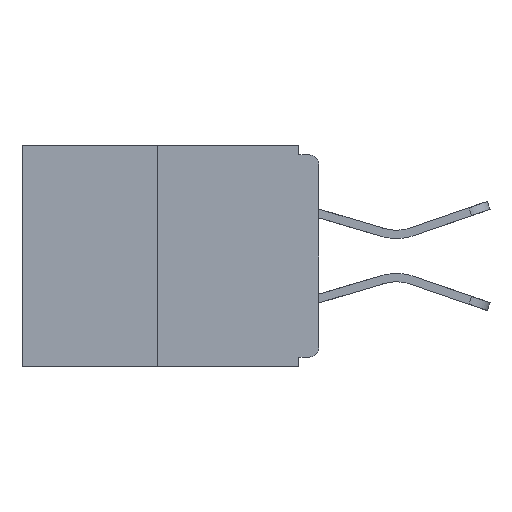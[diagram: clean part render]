
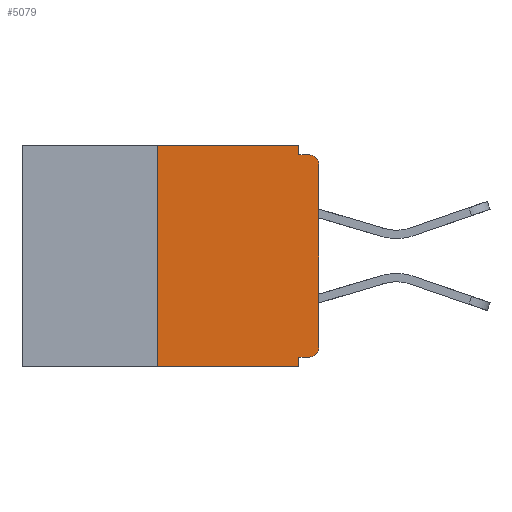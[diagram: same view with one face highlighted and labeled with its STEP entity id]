
A CAD part, left-side view. The second image highlights one B-rep face of the part: STEP entity #5079.
In plain terms, the highlighted planar face has unit normal (-1, 0, 0).
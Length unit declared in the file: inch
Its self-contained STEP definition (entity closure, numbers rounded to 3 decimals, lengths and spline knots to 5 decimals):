
#245 = DIRECTION ( 'NONE',  ( 1., 0., 0. ) ) ;
#256 = DIRECTION ( 'NONE',  ( -1., 0., 0. ) ) ;
#873 = VERTEX_POINT ( 'NONE', #2145 ) ;
#1524 = AXIS2_PLACEMENT_3D ( 'NONE', #5830, #245, #7463 ) ;
#1584 = LINE ( 'NONE', #21898, #17406 ) ;
#1611 = DIRECTION ( 'NONE',  ( 0., 0., 1. ) ) ;
#1694 = VERTEX_POINT ( 'NONE', #2825 ) ;
#2031 = CARTESIAN_POINT ( 'NONE',  ( 0., 0.015, -0.03 ) ) ;
#2145 = CARTESIAN_POINT ( 'NONE',  ( 0., 0., -0.03 ) ) ;
#2825 = CARTESIAN_POINT ( 'NONE',  ( 0., 0., -0.313 ) ) ;
#3088 = CARTESIAN_POINT ( 'NONE',  ( 0., 0.25, 0. ) ) ;
#3634 = VECTOR ( 'NONE', #22914, 39.37008 ) ;
#3731 = LINE ( 'NONE', #9060, #6418 ) ;
#3796 = EDGE_CURVE ( 'NONE', #4616, #9883, #1584, .T. ) ;
#3925 = PLANE ( 'NONE',  #1524 ) ;
#4080 = VECTOR ( 'NONE', #21179, 39.37008 ) ;
#4088 = VERTEX_POINT ( 'NONE', #3088 ) ;
#4372 = EDGE_CURVE ( 'NONE', #4088, #18091, #13389, .T. ) ;
#4557 = ORIENTED_EDGE ( 'NONE', *, *, #14546, .T. ) ;
#4616 = VERTEX_POINT ( 'NONE', #16344 ) ;
#4682 = AXIS2_PLACEMENT_3D ( 'NONE', #21091, #15497, #15159 ) ;
#4692 = DIRECTION ( 'NONE',  ( 0., -1., 0. ) ) ;
#4897 = CARTESIAN_POINT ( 'NONE',  ( 0., 0., 0. ) ) ;
#5079 = ADVANCED_FACE ( 'NONE', ( #19965 ), #3925, .F. ) ;
#5110 = CARTESIAN_POINT ( 'NONE',  ( 0., 0.031, 0. ) ) ;
#5830 = CARTESIAN_POINT ( 'NONE',  ( 0., 0.46, 0. ) ) ;
#6418 = VECTOR ( 'NONE', #1611, 39.37008 ) ;
#6474 = LINE ( 'NONE', #20983, #14541 ) ;
#6662 = CARTESIAN_POINT ( 'NONE',  ( 0., 0.015, -0.015 ) ) ;
#6881 = ORIENTED_EDGE ( 'NONE', *, *, #14597, .F. ) ;
#7301 = VECTOR ( 'NONE', #20868, 39.37008 ) ;
#7463 = DIRECTION ( 'NONE',  ( 0., 0., -1. ) ) ;
#7747 = VECTOR ( 'NONE', #17458, 39.37008 ) ;
#7790 = DIRECTION ( 'NONE',  ( 0., -1., 0. ) ) ;
#8229 = LINE ( 'NONE', #18727, #7301 ) ;
#8395 = CARTESIAN_POINT ( 'NONE',  ( 0., 0., -0.328 ) ) ;
#8791 = LINE ( 'NONE', #4897, #4080 ) ;
#9060 = CARTESIAN_POINT ( 'NONE',  ( 0., 0.25, 0. ) ) ;
#9267 = DIRECTION ( 'NONE',  ( 0., -1., 0. ) ) ;
#9642 = CARTESIAN_POINT ( 'NONE',  ( 0., 0.031, -0.343 ) ) ;
#9883 = VERTEX_POINT ( 'NONE', #9642 ) ;
#10383 = ORIENTED_EDGE ( 'NONE', *, *, #4372, .F. ) ;
#10672 = LINE ( 'NONE', #5110, #7747 ) ;
#10925 = DIRECTION ( 'NONE',  ( 0., 0., -1. ) ) ;
#10937 = EDGE_CURVE ( 'NONE', #4616, #4088, #3731, .T. ) ;
#11031 = AXIS2_PLACEMENT_3D ( 'NONE', #2031, #256, #10925 ) ;
#11621 = ORIENTED_EDGE ( 'NONE', *, *, #21747, .T. ) ;
#11745 = VERTEX_POINT ( 'NONE', #13734 ) ;
#12467 = EDGE_CURVE ( 'NONE', #873, #21868, #21676, .T. ) ;
#12709 = ORIENTED_EDGE ( 'NONE', *, *, #17196, .F. ) ;
#12951 = ORIENTED_EDGE ( 'NONE', *, *, #3796, .T. ) ;
#13389 = LINE ( 'NONE', #20652, #17081 ) ;
#13734 = CARTESIAN_POINT ( 'NONE',  ( 0., 0.031, -0.015 ) ) ;
#13936 = VERTEX_POINT ( 'NONE', #16734 ) ;
#14467 = EDGE_CURVE ( 'NONE', #17739, #9883, #8229, .T. ) ;
#14541 = VECTOR ( 'NONE', #4692, 39.37008 ) ;
#14546 = EDGE_CURVE ( 'NONE', #13936, #1694, #17572, .T. ) ;
#14597 = EDGE_CURVE ( 'NONE', #11745, #21868, #6474, .T. ) ;
#15159 = DIRECTION ( 'NONE',  ( 0., 0., -1. ) ) ;
#15497 = DIRECTION ( 'NONE',  ( -1., 0., 0. ) ) ;
#15771 = LINE ( 'NONE', #8395, #3634 ) ;
#15859 = ORIENTED_EDGE ( 'NONE', *, *, #18863, .F. ) ;
#16344 = CARTESIAN_POINT ( 'NONE',  ( 0., 0.25, -0.343 ) ) ;
#16734 = CARTESIAN_POINT ( 'NONE',  ( 0., 0.015, -0.328 ) ) ;
#17081 = VECTOR ( 'NONE', #7790, 39.37008 ) ;
#17196 = EDGE_CURVE ( 'NONE', #18091, #11745, #10672, .T. ) ;
#17404 = ORIENTED_EDGE ( 'NONE', *, *, #10937, .F. ) ;
#17406 = VECTOR ( 'NONE', #9267, 39.37008 ) ;
#17411 = CARTESIAN_POINT ( 'NONE',  ( 0., 0.031, 0. ) ) ;
#17458 = DIRECTION ( 'NONE',  ( 0., 0., -1. ) ) ;
#17572 = CIRCLE ( 'NONE', #4682, 0.015 ) ;
#17739 = VERTEX_POINT ( 'NONE', #19933 ) ;
#18091 = VERTEX_POINT ( 'NONE', #17411 ) ;
#18727 = CARTESIAN_POINT ( 'NONE',  ( 0., 0.031, -0.343 ) ) ;
#18863 = EDGE_CURVE ( 'NONE', #13936, #17739, #15771, .T. ) ;
#19933 = CARTESIAN_POINT ( 'NONE',  ( 0., 0.031, -0.328 ) ) ;
#19965 = FACE_OUTER_BOUND ( 'NONE', #23211, .T. ) ;
#20652 = CARTESIAN_POINT ( 'NONE',  ( 0., 0.46, 0. ) ) ;
#20868 = DIRECTION ( 'NONE',  ( 0., 0., -1. ) ) ;
#20891 = ORIENTED_EDGE ( 'NONE', *, *, #14467, .F. ) ;
#20983 = CARTESIAN_POINT ( 'NONE',  ( 0., 0., -0.015 ) ) ;
#21091 = CARTESIAN_POINT ( 'NONE',  ( 0., 0.015, -0.313 ) ) ;
#21179 = DIRECTION ( 'NONE',  ( 0., 0., 1. ) ) ;
#21676 = CIRCLE ( 'NONE', #11031, 0.015 ) ;
#21747 = EDGE_CURVE ( 'NONE', #1694, #873, #8791, .T. ) ;
#21868 = VERTEX_POINT ( 'NONE', #6662 ) ;
#21898 = CARTESIAN_POINT ( 'NONE',  ( 0., 0.46, -0.343 ) ) ;
#22914 = DIRECTION ( 'NONE',  ( 0., 1., 0. ) ) ;
#23211 = EDGE_LOOP ( 'NONE', ( #10383, #17404, #12951, #20891, #15859, #4557, #11621, #23358, #6881, #12709 ) ) ;
#23358 = ORIENTED_EDGE ( 'NONE', *, *, #12467, .T. ) ;
